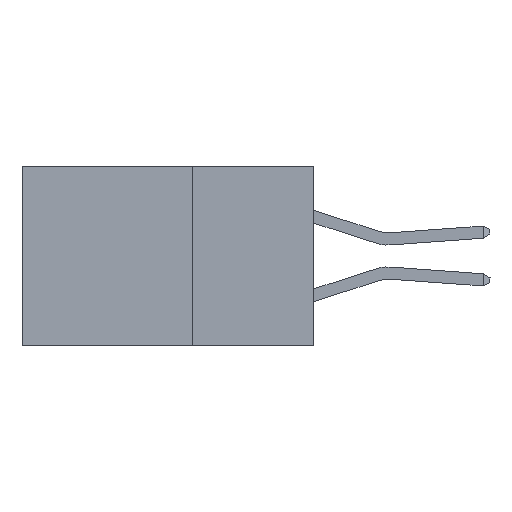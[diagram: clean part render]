
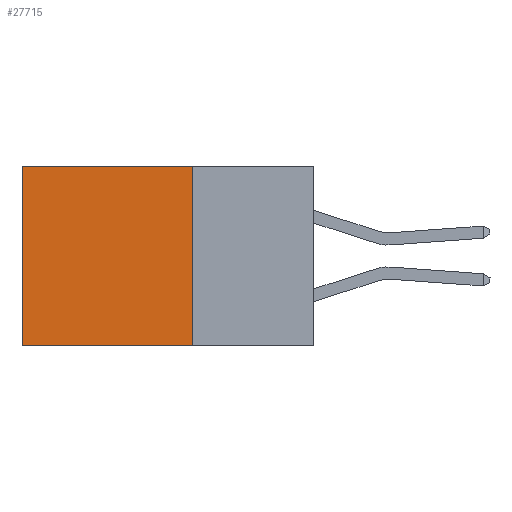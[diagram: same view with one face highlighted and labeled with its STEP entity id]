
A CAD part, left-side view. The second image highlights one B-rep face of the part: STEP entity #27715.
In plain terms, the highlighted planar face has unit normal (-1, 0, 0).
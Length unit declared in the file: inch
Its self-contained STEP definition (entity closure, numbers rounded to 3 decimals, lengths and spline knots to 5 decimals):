
#2501 = CARTESIAN_POINT ( 'NONE',  ( 0.2875, 0.6, 0. ) ) ;
#5001 = VECTOR ( 'NONE', #30411, 39.37008 ) ;
#6470 = CARTESIAN_POINT ( 'NONE',  ( 0.2875, 0.25, 0. ) ) ;
#8159 = EDGE_CURVE ( 'NONE', #20815, #10627, #26633, .T. ) ;
#9497 = VECTOR ( 'NONE', #25806, 39.37008 ) ;
#10627 = VERTEX_POINT ( 'NONE', #15134 ) ;
#11463 = DIRECTION ( 'NONE',  ( 0., 0., -1. ) ) ;
#11975 = LINE ( 'NONE', #21673, #26326 ) ;
#12415 = ORIENTED_EDGE ( 'NONE', *, *, #16594, .T. ) ;
#12677 = CARTESIAN_POINT ( 'NONE',  ( 0.2875, 0.25, -0.37 ) ) ;
#13045 = VERTEX_POINT ( 'NONE', #17921 ) ;
#13425 = CARTESIAN_POINT ( 'NONE',  ( 0.2875, 0.25, 0. ) ) ;
#15134 = CARTESIAN_POINT ( 'NONE',  ( 0.2875, 0.25, -0.37 ) ) ;
#16161 = CARTESIAN_POINT ( 'NONE',  ( 0.2875, 0.6, -0.37 ) ) ;
#16594 = EDGE_CURVE ( 'NONE', #20815, #13045, #11975, .T. ) ;
#16697 = LINE ( 'NONE', #2501, #30278 ) ;
#16792 = DIRECTION ( 'NONE',  ( 0., 1., 0. ) ) ;
#16811 = AXIS2_PLACEMENT_3D ( 'NONE', #6470, #21921, #11463 ) ;
#16954 = CARTESIAN_POINT ( 'NONE',  ( 0.2875, 0.25, 0. ) ) ;
#17336 = ORIENTED_EDGE ( 'NONE', *, *, #21627, .F. ) ;
#17921 = CARTESIAN_POINT ( 'NONE',  ( 0.2875, 0.6, 0. ) ) ;
#17950 = DIRECTION ( 'NONE',  ( 0., 0., -1. ) ) ;
#18136 = FACE_OUTER_BOUND ( 'NONE', #20805, .T. ) ;
#18209 = VERTEX_POINT ( 'NONE', #16161 ) ;
#18490 = LINE ( 'NONE', #12677, #5001 ) ;
#18588 = ORIENTED_EDGE ( 'NONE', *, *, #8159, .F. ) ;
#20805 = EDGE_LOOP ( 'NONE', ( #25920, #17336, #18588, #12415 ) ) ;
#20815 = VERTEX_POINT ( 'NONE', #16954 ) ;
#21627 = EDGE_CURVE ( 'NONE', #10627, #18209, #18490, .T. ) ;
#21673 = CARTESIAN_POINT ( 'NONE',  ( 0.2875, 0.25, 0. ) ) ;
#21701 = PLANE ( 'NONE',  #16811 ) ;
#21921 = DIRECTION ( 'NONE',  ( 1., 0., 0. ) ) ;
#25416 = EDGE_CURVE ( 'NONE', #13045, #18209, #16697, .T. ) ;
#25806 = DIRECTION ( 'NONE',  ( 0., 0., -1. ) ) ;
#25920 = ORIENTED_EDGE ( 'NONE', *, *, #25416, .T. ) ;
#26326 = VECTOR ( 'NONE', #16792, 39.37008 ) ;
#26633 = LINE ( 'NONE', #13425, #9497 ) ;
#27715 = ADVANCED_FACE ( 'NONE', ( #18136 ), #21701, .F. ) ;
#30278 = VECTOR ( 'NONE', #17950, 39.37008 ) ;
#30411 = DIRECTION ( 'NONE',  ( 0., 1., 0. ) ) ;
